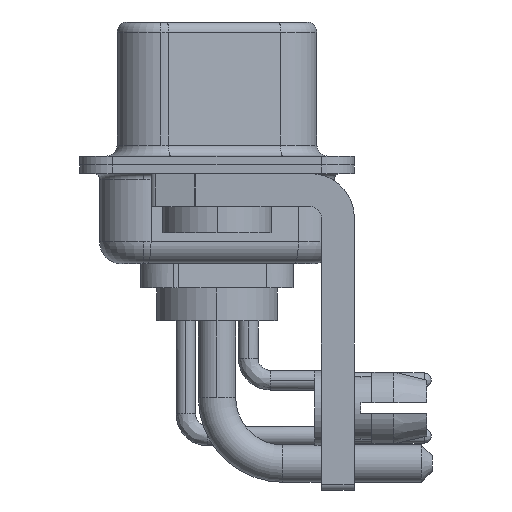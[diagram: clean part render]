
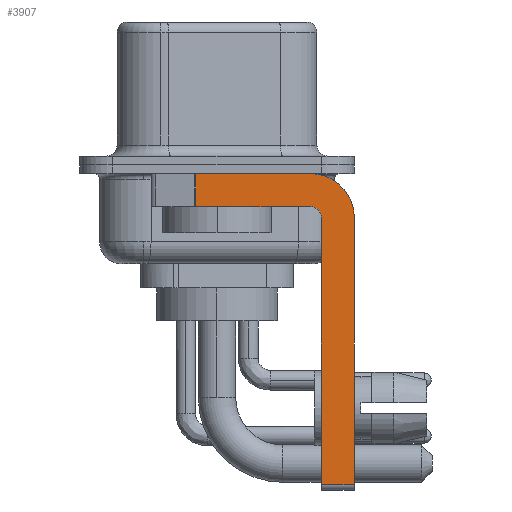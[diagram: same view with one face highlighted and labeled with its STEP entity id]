
A CAD part, left-side view. The second image highlights one B-rep face of the part: STEP entity #3907.
In plain terms, the highlighted planar face has unit normal (-1, 0, 0).
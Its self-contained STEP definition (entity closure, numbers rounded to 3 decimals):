
#550 = CARTESIAN_POINT ( 'NONE',  ( -2.9, -4.75, -14.8 ) ) ;
#679 = EDGE_CURVE ( 'NONE', #13578, #16343, #15763, .T. ) ;
#1670 = VERTEX_POINT ( 'NONE', #18299 ) ;
#1814 = DIRECTION ( 'NONE',  ( 1., 0., 0. ) ) ;
#2209 = AXIS2_PLACEMENT_3D ( 'NONE', #23422, #4681, #2618 ) ;
#2618 = DIRECTION ( 'NONE',  ( 0., 0., -1. ) ) ;
#2685 = EDGE_CURVE ( 'NONE', #16343, #11021, #9610, .T. ) ;
#2820 = DIRECTION ( 'NONE',  ( 0., 0., -1. ) ) ;
#3106 = CARTESIAN_POINT ( 'NONE',  ( -2.9, -6.25, -2.4 ) ) ;
#3907 = ADVANCED_FACE ( 'NONE', ( #20025 ), #14137, .F. ) ;
#3939 = ORIENTED_EDGE ( 'NONE', *, *, #9550, .F. ) ;
#4499 = CARTESIAN_POINT ( 'NONE',  ( -2.9, -4.25, -1.9 ) ) ;
#4681 = DIRECTION ( 'NONE',  ( 1., 0., 0. ) ) ;
#5484 = CARTESIAN_POINT ( 'NONE',  ( -2.9, -4.25, -14.55 ) ) ;
#5778 = DIRECTION ( 'NONE',  ( 0., 0., -1. ) ) ;
#5942 = DIRECTION ( 'NONE',  ( 0., 0., 1. ) ) ;
#5956 = VECTOR ( 'NONE', #24900, 1000. ) ;
#5977 = EDGE_CURVE ( 'NONE', #1670, #23647, #18966, .T. ) ;
#6020 = LINE ( 'NONE', #22992, #5956 ) ;
#6881 = ORIENTED_EDGE ( 'NONE', *, *, #679, .F. ) ;
#6967 = DIRECTION ( 'NONE',  ( 0., 0., 1. ) ) ;
#7058 = CARTESIAN_POINT ( 'NONE',  ( -2.9, -4.25, -0.4 ) ) ;
#8112 = DIRECTION ( 'NONE',  ( 0., 1., 0. ) ) ;
#8697 = LINE ( 'NONE', #15138, #25165 ) ;
#9545 = VECTOR ( 'NONE', #24368, 1000. ) ;
#9550 = EDGE_CURVE ( 'NONE', #15007, #13578, #6020, .T. ) ;
#9610 = LINE ( 'NONE', #26326, #14474 ) ;
#9996 = CARTESIAN_POINT ( 'NONE',  ( -2.9, -4.75, -14.55 ) ) ;
#11021 = VERTEX_POINT ( 'NONE', #23436 ) ;
#11913 = ORIENTED_EDGE ( 'NONE', *, *, #13334, .T. ) ;
#12955 = VECTOR ( 'NONE', #8112, 1000. ) ;
#13172 = ORIENTED_EDGE ( 'NONE', *, *, #5977, .F. ) ;
#13334 = EDGE_CURVE ( 'NONE', #17419, #11021, #26026, .T. ) ;
#13578 = VERTEX_POINT ( 'NONE', #7058 ) ;
#14137 = PLANE ( 'NONE',  #17205 ) ;
#14474 = VECTOR ( 'NONE', #5778, 1000. ) ;
#14886 = EDGE_CURVE ( 'NONE', #17419, #1670, #23532, .T. ) ;
#15007 = VERTEX_POINT ( 'NONE', #24469 ) ;
#15138 = CARTESIAN_POINT ( 'NONE',  ( -2.9, 0.978, -1.9 ) ) ;
#15252 = CARTESIAN_POINT ( 'NONE',  ( -2.9, 0.978, -1.9 ) ) ;
#15466 = ORIENTED_EDGE ( 'NONE', *, *, #14886, .F. ) ;
#15763 = CIRCLE ( 'NONE', #2209, 2. ) ;
#16198 = CARTESIAN_POINT ( 'NONE',  ( -2.9, -4.25, -2.4 ) ) ;
#16343 = VERTEX_POINT ( 'NONE', #3106 ) ;
#16757 = CARTESIAN_POINT ( 'NONE',  ( -2.9, -4.25, -2.4 ) ) ;
#17205 = AXIS2_PLACEMENT_3D ( 'NONE', #16198, #1814, #24794 ) ;
#17419 = VERTEX_POINT ( 'NONE', #9996 ) ;
#18003 = ORIENTED_EDGE ( 'NONE', *, *, #26016, .T. ) ;
#18299 = CARTESIAN_POINT ( 'NONE',  ( -2.9, -4.75, -2.4 ) ) ;
#18658 = DIRECTION ( 'NONE',  ( -1., 0., 0. ) ) ;
#18966 = CIRCLE ( 'NONE', #25103, 0.5 ) ;
#20025 = FACE_OUTER_BOUND ( 'NONE', #20330, .T. ) ;
#20330 = EDGE_LOOP ( 'NONE', ( #3939, #18003, #26756, #13172, #15466, #11913, #20953, #6881 ) ) ;
#20953 = ORIENTED_EDGE ( 'NONE', *, *, #2685, .F. ) ;
#21044 = VERTEX_POINT ( 'NONE', #15252 ) ;
#22992 = CARTESIAN_POINT ( 'NONE',  ( -2.9, 3., -0.4 ) ) ;
#23422 = CARTESIAN_POINT ( 'NONE',  ( -2.9, -4.25, -2.4 ) ) ;
#23436 = CARTESIAN_POINT ( 'NONE',  ( -2.9, -6.25, -14.55 ) ) ;
#23532 = LINE ( 'NONE', #550, #25351 ) ;
#23647 = VERTEX_POINT ( 'NONE', #4499 ) ;
#24368 = DIRECTION ( 'NONE',  ( 0., -1., 0. ) ) ;
#24469 = CARTESIAN_POINT ( 'NONE',  ( -2.9, 0.978, -0.4 ) ) ;
#24685 = LINE ( 'NONE', #26884, #12955 ) ;
#24794 = DIRECTION ( 'NONE',  ( 0., 0., -1. ) ) ;
#24900 = DIRECTION ( 'NONE',  ( 0., -1., 0. ) ) ;
#25103 = AXIS2_PLACEMENT_3D ( 'NONE', #16757, #18658, #5942 ) ;
#25165 = VECTOR ( 'NONE', #2820, 1000. ) ;
#25351 = VECTOR ( 'NONE', #6967, 1000. ) ;
#26016 = EDGE_CURVE ( 'NONE', #15007, #21044, #8697, .T. ) ;
#26026 = LINE ( 'NONE', #5484, #9545 ) ;
#26326 = CARTESIAN_POINT ( 'NONE',  ( -2.9, -6.25, -2.4 ) ) ;
#26452 = EDGE_CURVE ( 'NONE', #23647, #21044, #24685, .T. ) ;
#26756 = ORIENTED_EDGE ( 'NONE', *, *, #26452, .F. ) ;
#26884 = CARTESIAN_POINT ( 'NONE',  ( -2.9, -4.25, -1.9 ) ) ;
